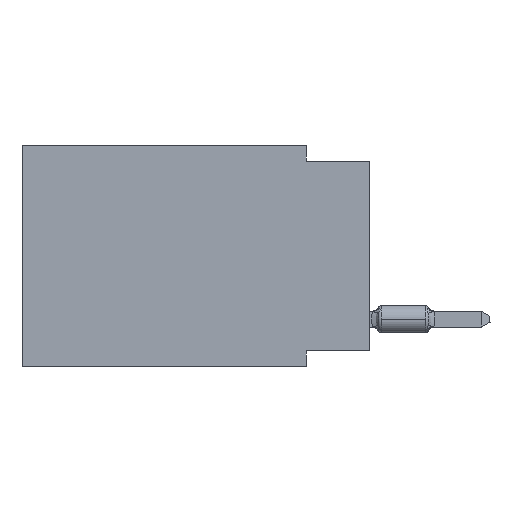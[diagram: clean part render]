
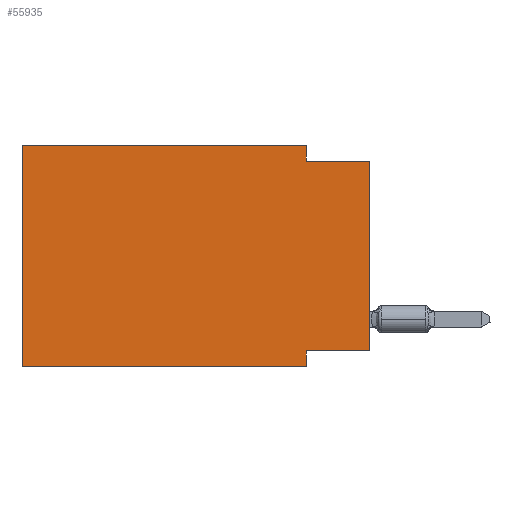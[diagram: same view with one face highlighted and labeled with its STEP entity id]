
A CAD part, left-side view. The second image highlights one B-rep face of the part: STEP entity #55935.
In plain terms, the highlighted planar face has unit normal (-1, 0, 0).
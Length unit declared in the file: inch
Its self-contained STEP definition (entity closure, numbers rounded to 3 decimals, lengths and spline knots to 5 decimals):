
#1377 = CARTESIAN_POINT ( 'NONE',  ( 0., 0.1, 0. ) ) ;
#2819 = EDGE_CURVE ( 'NONE', #64616, #41125, #19703, .T. ) ;
#5309 = ORIENTED_EDGE ( 'NONE', *, *, #2819, .T. ) ;
#5472 = VERTEX_POINT ( 'NONE', #16337 ) ;
#6031 = DIRECTION ( 'NONE',  ( 0., 1., 0. ) ) ;
#7120 = EDGE_CURVE ( 'NONE', #61136, #23901, #34255, .T. ) ;
#7869 = LINE ( 'NONE', #67439, #12872 ) ;
#8532 = EDGE_CURVE ( 'NONE', #5472, #27865, #52752, .T. ) ;
#8564 = CARTESIAN_POINT ( 'NONE',  ( 0., 0.55, -0.35 ) ) ;
#9314 = ORIENTED_EDGE ( 'NONE', *, *, #8532, .F. ) ;
#9524 = VECTOR ( 'NONE', #11893, 39.37008 ) ;
#9717 = CARTESIAN_POINT ( 'NONE',  ( 0., 0.1, -0.35 ) ) ;
#11893 = DIRECTION ( 'NONE',  ( 0., -1., 0. ) ) ;
#12312 = EDGE_CURVE ( 'NONE', #64616, #5472, #55749, .T. ) ;
#12872 = VECTOR ( 'NONE', #6031, 39.37008 ) ;
#13184 = CARTESIAN_POINT ( 'NONE',  ( 0., 0.55, 0. ) ) ;
#13556 = CARTESIAN_POINT ( 'NONE',  ( 0., 0.55, 0. ) ) ;
#16337 = CARTESIAN_POINT ( 'NONE',  ( 0., 0.55, 0. ) ) ;
#17448 = CARTESIAN_POINT ( 'NONE',  ( 0., 0., -0.025 ) ) ;
#17518 = ORIENTED_EDGE ( 'NONE', *, *, #31677, .F. ) ;
#18332 = CARTESIAN_POINT ( 'NONE',  ( 0., 0.55, -0.35 ) ) ;
#18354 = LINE ( 'NONE', #19038, #57630 ) ;
#18583 = CARTESIAN_POINT ( 'NONE',  ( 0., 0.1, -0.325 ) ) ;
#19038 = CARTESIAN_POINT ( 'NONE',  ( 0., 0., 0. ) ) ;
#19703 = LINE ( 'NONE', #18332, #48420 ) ;
#23277 = DIRECTION ( 'NONE',  ( 0., -1., 0. ) ) ;
#23621 = VECTOR ( 'NONE', #23277, 39.37008 ) ;
#23830 = DIRECTION ( 'NONE',  ( 0., 0., -1. ) ) ;
#23901 = VERTEX_POINT ( 'NONE', #44876 ) ;
#24444 = EDGE_CURVE ( 'NONE', #37535, #23901, #18354, .T. ) ;
#25504 = AXIS2_PLACEMENT_3D ( 'NONE', #13184, #45782, #23830 ) ;
#27153 = ORIENTED_EDGE ( 'NONE', *, *, #24444, .T. ) ;
#27186 = VECTOR ( 'NONE', #59670, 39.37008 ) ;
#27210 = ORIENTED_EDGE ( 'NONE', *, *, #7120, .F. ) ;
#27865 = VERTEX_POINT ( 'NONE', #42926 ) ;
#28662 = DIRECTION ( 'NONE',  ( 0., 0., 1. ) ) ;
#29657 = PLANE ( 'NONE',  #25504 ) ;
#31677 = EDGE_CURVE ( 'NONE', #49271, #41125, #38783, .T. ) ;
#34255 = LINE ( 'NONE', #17448, #23621 ) ;
#36744 = CARTESIAN_POINT ( 'NONE',  ( 0., 0., -0.325 ) ) ;
#36974 = ORIENTED_EDGE ( 'NONE', *, *, #63435, .F. ) ;
#37535 = VERTEX_POINT ( 'NONE', #36744 ) ;
#38000 = CARTESIAN_POINT ( 'NONE',  ( 0., 0.55, 0. ) ) ;
#38783 = LINE ( 'NONE', #65151, #47980 ) ;
#39125 = DIRECTION ( 'NONE',  ( 0., 0., -1. ) ) ;
#39300 = DIRECTION ( 'NONE',  ( 0., 0., 1. ) ) ;
#41125 = VERTEX_POINT ( 'NONE', #9717 ) ;
#42578 = LINE ( 'NONE', #1377, #27186 ) ;
#42926 = CARTESIAN_POINT ( 'NONE',  ( 0., 0.1, 0. ) ) ;
#44876 = CARTESIAN_POINT ( 'NONE',  ( 0., 0., -0.025 ) ) ;
#45782 = DIRECTION ( 'NONE',  ( 1., 0., 0. ) ) ;
#47980 = VECTOR ( 'NONE', #39125, 39.37008 ) ;
#48420 = VECTOR ( 'NONE', #56057, 39.37008 ) ;
#49271 = VERTEX_POINT ( 'NONE', #18583 ) ;
#51324 = CARTESIAN_POINT ( 'NONE',  ( 0., 0.1, -0.025 ) ) ;
#52752 = LINE ( 'NONE', #38000, #9524 ) ;
#55749 = LINE ( 'NONE', #13556, #60295 ) ;
#55935 = ADVANCED_FACE ( 'NONE', ( #65306 ), #29657, .F. ) ;
#56057 = DIRECTION ( 'NONE',  ( 0., -1., 0. ) ) ;
#57183 = ORIENTED_EDGE ( 'NONE', *, *, #12312, .F. ) ;
#57630 = VECTOR ( 'NONE', #39300, 39.37008 ) ;
#59670 = DIRECTION ( 'NONE',  ( 0., 0., -1. ) ) ;
#60295 = VECTOR ( 'NONE', #28662, 39.37008 ) ;
#61136 = VERTEX_POINT ( 'NONE', #51324 ) ;
#61944 = ORIENTED_EDGE ( 'NONE', *, *, #64575, .F. ) ;
#63435 = EDGE_CURVE ( 'NONE', #37535, #49271, #7869, .T. ) ;
#64575 = EDGE_CURVE ( 'NONE', #27865, #61136, #42578, .T. ) ;
#64616 = VERTEX_POINT ( 'NONE', #8564 ) ;
#65151 = CARTESIAN_POINT ( 'NONE',  ( 0., 0.1, -0.35 ) ) ;
#65306 = FACE_OUTER_BOUND ( 'NONE', #65345, .T. ) ;
#65345 = EDGE_LOOP ( 'NONE', ( #27153, #27210, #61944, #9314, #57183, #5309, #17518, #36974 ) ) ;
#67439 = CARTESIAN_POINT ( 'NONE',  ( 0., 0., -0.325 ) ) ;
